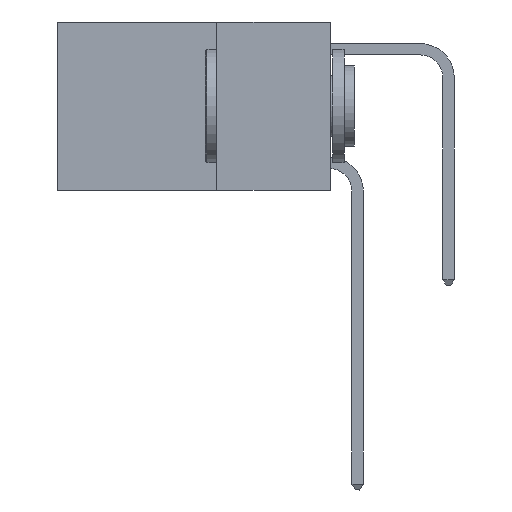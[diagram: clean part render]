
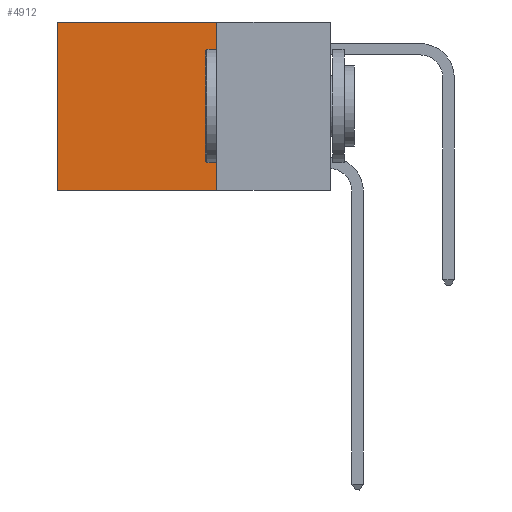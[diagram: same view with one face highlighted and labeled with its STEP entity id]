
A CAD part, left-side view. The second image highlights one B-rep face of the part: STEP entity #4912.
In plain terms, the highlighted planar face has unit normal (-1, 0, 0).
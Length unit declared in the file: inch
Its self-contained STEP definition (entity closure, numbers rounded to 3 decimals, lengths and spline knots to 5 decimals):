
#740 = CARTESIAN_POINT ( 'NONE',  ( 0.2625, 0.25, 0. ) ) ;
#1540 = DIRECTION ( 'NONE',  ( 0., 1., 0. ) ) ;
#2233 = PLANE ( 'NONE',  #24282 ) ;
#2400 = CARTESIAN_POINT ( 'NONE',  ( 0.2625, 0.25, 0. ) ) ;
#2526 = CARTESIAN_POINT ( 'NONE',  ( 0.2625, 0.25, 0. ) ) ;
#2782 = EDGE_CURVE ( 'NONE', #4391, #17101, #15601, .T. ) ;
#3804 = VECTOR ( 'NONE', #17396, 39.37008 ) ;
#4391 = VERTEX_POINT ( 'NONE', #2526 ) ;
#4912 = ADVANCED_FACE ( 'NONE', ( #13402 ), #2233, .F. ) ;
#5148 = EDGE_LOOP ( 'NONE', ( #9989, #18864, #11895, #24823 ) ) ;
#6946 = EDGE_CURVE ( 'NONE', #4391, #19400, #18637, .T. ) ;
#7208 = LINE ( 'NONE', #9424, #9565 ) ;
#7261 = DIRECTION ( 'NONE',  ( 0., 1., 0. ) ) ;
#9424 = CARTESIAN_POINT ( 'NONE',  ( 0.2625, 0.25, -0.37 ) ) ;
#9565 = VECTOR ( 'NONE', #7261, 39.37008 ) ;
#9965 = VECTOR ( 'NONE', #1540, 39.37008 ) ;
#9989 = ORIENTED_EDGE ( 'NONE', *, *, #24179, .T. ) ;
#11848 = VERTEX_POINT ( 'NONE', #25706 ) ;
#11895 = ORIENTED_EDGE ( 'NONE', *, *, #6946, .F. ) ;
#13402 = FACE_OUTER_BOUND ( 'NONE', #5148, .T. ) ;
#15601 = LINE ( 'NONE', #27152, #9965 ) ;
#15848 = DIRECTION ( 'NONE',  ( 0., 0., -1. ) ) ;
#17101 = VERTEX_POINT ( 'NONE', #17882 ) ;
#17396 = DIRECTION ( 'NONE',  ( 0., 0., -1. ) ) ;
#17816 = CARTESIAN_POINT ( 'NONE',  ( 0.2625, 0.6, 0. ) ) ;
#17882 = CARTESIAN_POINT ( 'NONE',  ( 0.2625, 0.6, 0. ) ) ;
#18402 = LINE ( 'NONE', #17816, #21697 ) ;
#18637 = LINE ( 'NONE', #2400, #3804 ) ;
#18864 = ORIENTED_EDGE ( 'NONE', *, *, #25747, .F. ) ;
#19400 = VERTEX_POINT ( 'NONE', #23462 ) ;
#21697 = VECTOR ( 'NONE', #26360, 39.37008 ) ;
#23462 = CARTESIAN_POINT ( 'NONE',  ( 0.2625, 0.25, -0.37 ) ) ;
#24179 = EDGE_CURVE ( 'NONE', #17101, #11848, #18402, .T. ) ;
#24282 = AXIS2_PLACEMENT_3D ( 'NONE', #740, #26528, #15848 ) ;
#24823 = ORIENTED_EDGE ( 'NONE', *, *, #2782, .T. ) ;
#25706 = CARTESIAN_POINT ( 'NONE',  ( 0.2625, 0.6, -0.37 ) ) ;
#25747 = EDGE_CURVE ( 'NONE', #19400, #11848, #7208, .T. ) ;
#26360 = DIRECTION ( 'NONE',  ( 0., 0., -1. ) ) ;
#26528 = DIRECTION ( 'NONE',  ( 1., 0., 0. ) ) ;
#27152 = CARTESIAN_POINT ( 'NONE',  ( 0.2625, 0.25, 0. ) ) ;
